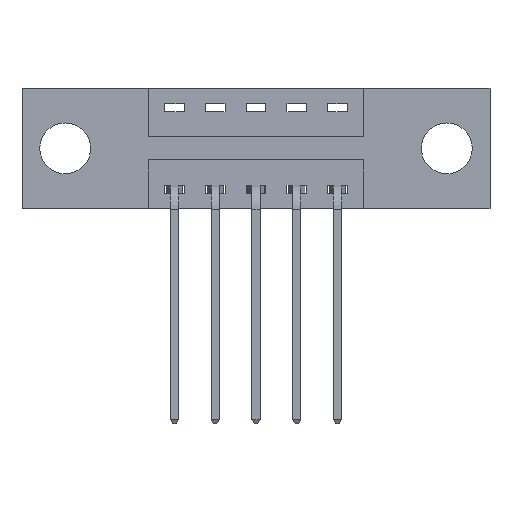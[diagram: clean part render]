
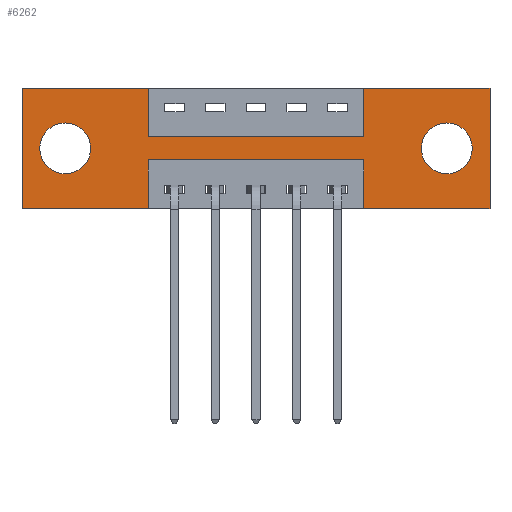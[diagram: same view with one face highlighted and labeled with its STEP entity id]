
A CAD part, front view. The second image highlights one B-rep face of the part: STEP entity #6262.
In plain terms, the highlighted planar face has unit normal (0, -1, 0).
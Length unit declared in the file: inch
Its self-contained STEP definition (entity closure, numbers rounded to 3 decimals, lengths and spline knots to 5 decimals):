
#17 = CARTESIAN_POINT ( 'NONE',  ( 1.3025, 0., -0.107 ) ) ;
#54 = AXIS2_PLACEMENT_3D ( 'NONE', #6915, #5585, #8227 ) ;
#188 = CARTESIAN_POINT ( 'NONE',  ( 0.1325, 0., -0.263 ) ) ;
#190 = DIRECTION ( 'NONE',  ( 1., 0., 0. ) ) ;
#232 = FACE_BOUND ( 'NONE', #7393, .T. ) ;
#237 = ORIENTED_EDGE ( 'NONE', *, *, #1024, .F. ) ;
#328 = VECTOR ( 'NONE', #3178, 39.37008 ) ;
#433 = AXIS2_PLACEMENT_3D ( 'NONE', #8575, #2546, #1128 ) ;
#530 = CARTESIAN_POINT ( 'NONE',  ( 0.3875, 0., -0.22 ) ) ;
#536 = VERTEX_POINT ( 'NONE', #3604 ) ;
#569 = CARTESIAN_POINT ( 'NONE',  ( 1.3025, 0., -0.263 ) ) ;
#656 = CARTESIAN_POINT ( 'NONE',  ( 0., 0., -0.37 ) ) ;
#726 = CARTESIAN_POINT ( 'NONE',  ( 0., 0., 0. ) ) ;
#883 = VERTEX_POINT ( 'NONE', #4192 ) ;
#1024 = EDGE_CURVE ( 'NONE', #5832, #7851, #3753, .T. ) ;
#1026 = DIRECTION ( 'NONE',  ( 1., 0., 0. ) ) ;
#1094 = VECTOR ( 'NONE', #5826, 39.37008 ) ;
#1128 = DIRECTION ( 'NONE',  ( 0., 0., -1. ) ) ;
#1164 = ORIENTED_EDGE ( 'NONE', *, *, #1781, .F. ) ;
#1369 = VERTEX_POINT ( 'NONE', #8116 ) ;
#1379 = CIRCLE ( 'NONE', #8172, 0.078 ) ;
#1431 = VERTEX_POINT ( 'NONE', #7352 ) ;
#1594 = EDGE_CURVE ( 'NONE', #6373, #5877, #1379, .T. ) ;
#1678 = EDGE_CURVE ( 'NONE', #6737, #4426, #6624, .T. ) ;
#1781 = EDGE_CURVE ( 'NONE', #7318, #1431, #6485, .T. ) ;
#1797 = EDGE_CURVE ( 'NONE', #536, #1929, #1943, .T. ) ;
#1811 = DIRECTION ( 'NONE',  ( 0., 0., -1. ) ) ;
#1915 = ORIENTED_EDGE ( 'NONE', *, *, #2250, .F. ) ;
#1919 = VECTOR ( 'NONE', #6893, 39.37008 ) ;
#1924 = DIRECTION ( 'NONE',  ( 0., 1., 0. ) ) ;
#1929 = VERTEX_POINT ( 'NONE', #4939 ) ;
#1943 = LINE ( 'NONE', #3938, #5810 ) ;
#1967 = CARTESIAN_POINT ( 'NONE',  ( 0., 0., -0.37 ) ) ;
#2059 = CARTESIAN_POINT ( 'NONE',  ( 1.0475, 0., -0.15 ) ) ;
#2137 = CARTESIAN_POINT ( 'NONE',  ( 0.1325, 0., -0.185 ) ) ;
#2245 = ORIENTED_EDGE ( 'NONE', *, *, #5394, .F. ) ;
#2250 = EDGE_CURVE ( 'NONE', #1929, #5832, #4878, .T. ) ;
#2258 = ORIENTED_EDGE ( 'NONE', *, *, #5961, .F. ) ;
#2279 = PLANE ( 'NONE',  #54 ) ;
#2301 = CIRCLE ( 'NONE', #2452, 0.078 ) ;
#2338 = VERTEX_POINT ( 'NONE', #4967 ) ;
#2349 = CARTESIAN_POINT ( 'NONE',  ( 0., 0., 0. ) ) ;
#2377 = VERTEX_POINT ( 'NONE', #569 ) ;
#2452 = AXIS2_PLACEMENT_3D ( 'NONE', #5189, #1924, #4547 ) ;
#2518 = VERTEX_POINT ( 'NONE', #17 ) ;
#2521 = LINE ( 'NONE', #4608, #328 ) ;
#2543 = LINE ( 'NONE', #1967, #6889 ) ;
#2546 = DIRECTION ( 'NONE',  ( 0., 1., 0. ) ) ;
#2562 = CARTESIAN_POINT ( 'NONE',  ( 0.3875, 0., -0.37 ) ) ;
#2706 = ORIENTED_EDGE ( 'NONE', *, *, #1594, .T. ) ;
#2849 = VECTOR ( 'NONE', #1026, 39.37008 ) ;
#2943 = LINE ( 'NONE', #4194, #1919 ) ;
#3178 = DIRECTION ( 'NONE',  ( 0., 0., 1. ) ) ;
#3236 = DIRECTION ( 'NONE',  ( -1., 0., 0. ) ) ;
#3291 = DIRECTION ( 'NONE',  ( 0., 0., 1. ) ) ;
#3447 = AXIS2_PLACEMENT_3D ( 'NONE', #5946, #5445, #6814 ) ;
#3466 = ORIENTED_EDGE ( 'NONE', *, *, #7382, .F. ) ;
#3604 = CARTESIAN_POINT ( 'NONE',  ( 0.3875, 0., 0. ) ) ;
#3627 = ORIENTED_EDGE ( 'NONE', *, *, #7746, .F. ) ;
#3714 = CIRCLE ( 'NONE', #3447, 0.078 ) ;
#3753 = LINE ( 'NONE', #6382, #6513 ) ;
#3861 = EDGE_LOOP ( 'NONE', ( #7872, #2706 ) ) ;
#3938 = CARTESIAN_POINT ( 'NONE',  ( 0.3875, 0., 0. ) ) ;
#3940 = CIRCLE ( 'NONE', #433, 0.078 ) ;
#4048 = VECTOR ( 'NONE', #8064, 39.37008 ) ;
#4192 = CARTESIAN_POINT ( 'NONE',  ( 1.435, 0., 0. ) ) ;
#4194 = CARTESIAN_POINT ( 'NONE',  ( 1.435, 0., 0. ) ) ;
#4196 = CARTESIAN_POINT ( 'NONE',  ( 1.0475, 0., 0. ) ) ;
#4205 = ORIENTED_EDGE ( 'NONE', *, *, #1678, .F. ) ;
#4236 = VECTOR ( 'NONE', #8556, 39.37008 ) ;
#4306 = VECTOR ( 'NONE', #5950, 39.37008 ) ;
#4426 = VERTEX_POINT ( 'NONE', #656 ) ;
#4547 = DIRECTION ( 'NONE',  ( 0., 0., 1. ) ) ;
#4608 = CARTESIAN_POINT ( 'NONE',  ( 0., 0., 0. ) ) ;
#4680 = ORIENTED_EDGE ( 'NONE', *, *, #6818, .F. ) ;
#4761 = DIRECTION ( 'NONE',  ( 0., 1., 0. ) ) ;
#4859 = ORIENTED_EDGE ( 'NONE', *, *, #5351, .T. ) ;
#4878 = LINE ( 'NONE', #6824, #4048 ) ;
#4939 = CARTESIAN_POINT ( 'NONE',  ( 0.3875, 0., -0.15 ) ) ;
#4967 = CARTESIAN_POINT ( 'NONE',  ( 0.3875, 0., -0.22 ) ) ;
#5067 = DIRECTION ( 'NONE',  ( 0., 0., 1. ) ) ;
#5131 = LINE ( 'NONE', #530, #1094 ) ;
#5189 = CARTESIAN_POINT ( 'NONE',  ( 0.1325, 0., -0.185 ) ) ;
#5272 = CARTESIAN_POINT ( 'NONE',  ( 1.0475, 0., -0.37 ) ) ;
#5351 = EDGE_CURVE ( 'NONE', #2518, #2377, #3940, .T. ) ;
#5394 = EDGE_CURVE ( 'NONE', #7851, #883, #5420, .T. ) ;
#5420 = LINE ( 'NONE', #726, #5572 ) ;
#5445 = DIRECTION ( 'NONE',  ( 0., 1., 0. ) ) ;
#5548 = VERTEX_POINT ( 'NONE', #8480 ) ;
#5572 = VECTOR ( 'NONE', #190, 39.37008 ) ;
#5585 = DIRECTION ( 'NONE',  ( 0., -1., 0. ) ) ;
#5677 = VECTOR ( 'NONE', #3291, 39.37008 ) ;
#5736 = LINE ( 'NONE', #2562, #4236 ) ;
#5810 = VECTOR ( 'NONE', #1811, 39.37008 ) ;
#5826 = DIRECTION ( 'NONE',  ( -1., 0., 0. ) ) ;
#5832 = VERTEX_POINT ( 'NONE', #2059 ) ;
#5877 = VERTEX_POINT ( 'NONE', #8442 ) ;
#5946 = CARTESIAN_POINT ( 'NONE',  ( 1.3025, 0., -0.185 ) ) ;
#5950 = DIRECTION ( 'NONE',  ( -1., 0., 0. ) ) ;
#5961 = EDGE_CURVE ( 'NONE', #2338, #6737, #5736, .T. ) ;
#6262 = ADVANCED_FACE ( 'NONE', ( #232, #6964, #8189 ), #2279, .T. ) ;
#6312 = EDGE_CURVE ( 'NONE', #5877, #6373, #2301, .T. ) ;
#6373 = VERTEX_POINT ( 'NONE', #188 ) ;
#6382 = CARTESIAN_POINT ( 'NONE',  ( 1.0475, 0., 0. ) ) ;
#6439 = EDGE_CURVE ( 'NONE', #5548, #536, #6951, .T. ) ;
#6485 = LINE ( 'NONE', #7195, #5677 ) ;
#6513 = VECTOR ( 'NONE', #5067, 39.37008 ) ;
#6624 = LINE ( 'NONE', #7412, #4306 ) ;
#6670 = EDGE_CURVE ( 'NONE', #1369, #7318, #2543, .T. ) ;
#6737 = VERTEX_POINT ( 'NONE', #8399 ) ;
#6814 = DIRECTION ( 'NONE',  ( 0., 0., -1. ) ) ;
#6818 = EDGE_CURVE ( 'NONE', #4426, #5548, #2521, .T. ) ;
#6824 = CARTESIAN_POINT ( 'NONE',  ( 0.3875, 0., -0.15 ) ) ;
#6883 = ORIENTED_EDGE ( 'NONE', *, *, #1797, .F. ) ;
#6889 = VECTOR ( 'NONE', #3236, 39.37008 ) ;
#6893 = DIRECTION ( 'NONE',  ( 0., 0., -1. ) ) ;
#6915 = CARTESIAN_POINT ( 'NONE',  ( 0., 0., -0.37 ) ) ;
#6951 = LINE ( 'NONE', #2349, #2849 ) ;
#6964 = FACE_BOUND ( 'NONE', #3861, .T. ) ;
#7195 = CARTESIAN_POINT ( 'NONE',  ( 1.0475, 0., -0.37 ) ) ;
#7283 = ORIENTED_EDGE ( 'NONE', *, *, #6670, .F. ) ;
#7318 = VERTEX_POINT ( 'NONE', #5272 ) ;
#7331 = EDGE_LOOP ( 'NONE', ( #2258, #3627, #1164, #7283, #3466, #2245, #237, #1915, #6883, #7357, #4680, #4205 ) ) ;
#7352 = CARTESIAN_POINT ( 'NONE',  ( 1.0475, 0., -0.22 ) ) ;
#7357 = ORIENTED_EDGE ( 'NONE', *, *, #6439, .F. ) ;
#7382 = EDGE_CURVE ( 'NONE', #883, #1369, #2943, .T. ) ;
#7393 = EDGE_LOOP ( 'NONE', ( #4859, #8526 ) ) ;
#7412 = CARTESIAN_POINT ( 'NONE',  ( 0., 0., -0.37 ) ) ;
#7430 = DIRECTION ( 'NONE',  ( 0., 0., 1. ) ) ;
#7746 = EDGE_CURVE ( 'NONE', #1431, #2338, #5131, .T. ) ;
#7800 = EDGE_CURVE ( 'NONE', #2377, #2518, #3714, .T. ) ;
#7851 = VERTEX_POINT ( 'NONE', #4196 ) ;
#7872 = ORIENTED_EDGE ( 'NONE', *, *, #6312, .T. ) ;
#8064 = DIRECTION ( 'NONE',  ( 1., 0., 0. ) ) ;
#8116 = CARTESIAN_POINT ( 'NONE',  ( 1.435, 0., -0.37 ) ) ;
#8172 = AXIS2_PLACEMENT_3D ( 'NONE', #2137, #4761, #7430 ) ;
#8189 = FACE_OUTER_BOUND ( 'NONE', #7331, .T. ) ;
#8227 = DIRECTION ( 'NONE',  ( 0., 0., -1. ) ) ;
#8399 = CARTESIAN_POINT ( 'NONE',  ( 0.3875, 0., -0.37 ) ) ;
#8442 = CARTESIAN_POINT ( 'NONE',  ( 0.1325, 0., -0.107 ) ) ;
#8480 = CARTESIAN_POINT ( 'NONE',  ( 0., 0., 0. ) ) ;
#8526 = ORIENTED_EDGE ( 'NONE', *, *, #7800, .T. ) ;
#8556 = DIRECTION ( 'NONE',  ( 0., 0., -1. ) ) ;
#8575 = CARTESIAN_POINT ( 'NONE',  ( 1.3025, 0., -0.185 ) ) ;
